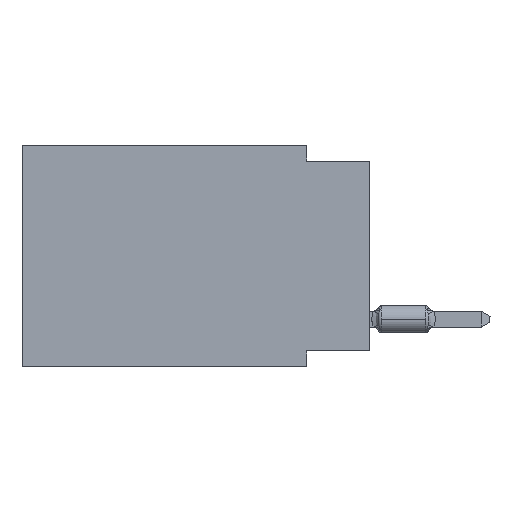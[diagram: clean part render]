
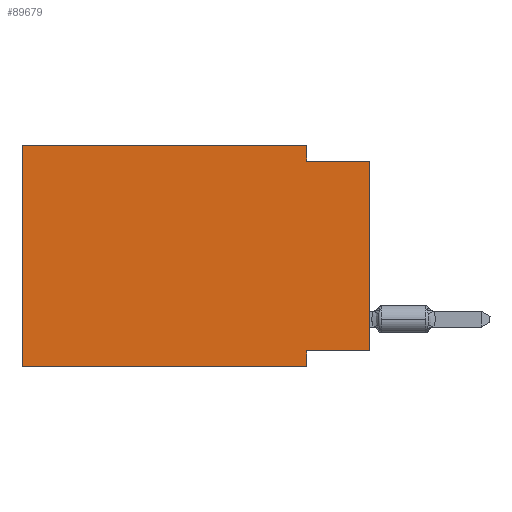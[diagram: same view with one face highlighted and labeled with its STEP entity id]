
A CAD part, left-side view. The second image highlights one B-rep face of the part: STEP entity #89679.
In plain terms, the highlighted planar face has unit normal (-1, 0, 0).
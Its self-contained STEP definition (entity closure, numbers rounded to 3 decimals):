
#3311 = CARTESIAN_POINT ( 'NONE',  ( 0., 2.54, -8.89 ) ) ;
#4840 = CARTESIAN_POINT ( 'NONE',  ( 0., 0., -0.635 ) ) ;
#7582 = PLANE ( 'NONE',  #13161 ) ;
#9186 = ORIENTED_EDGE ( 'NONE', *, *, #81791, .T. ) ;
#12275 = LINE ( 'NONE', #12768, #88802 ) ;
#12284 = DIRECTION ( 'NONE',  ( 0., 0., 1. ) ) ;
#12288 = DIRECTION ( 'NONE',  ( 0., -1., 0. ) ) ;
#12687 = EDGE_LOOP ( 'NONE', ( #56744, #20710, #52912, #78316, #48827, #9186, #57996, #62685 ) ) ;
#12768 = CARTESIAN_POINT ( 'NONE',  ( 0., 2.54, 0. ) ) ;
#13161 = AXIS2_PLACEMENT_3D ( 'NONE', #30740, #92196, #77064 ) ;
#14681 = CARTESIAN_POINT ( 'NONE',  ( 0., 2.54, -8.89 ) ) ;
#15447 = DIRECTION ( 'NONE',  ( 0., 0., 1. ) ) ;
#17630 = EDGE_CURVE ( 'NONE', #24997, #32959, #20441, .T. ) ;
#19634 = CARTESIAN_POINT ( 'NONE',  ( 0., 2.54, -8.255 ) ) ;
#20353 = LINE ( 'NONE', #60130, #80948 ) ;
#20441 = LINE ( 'NONE', #4840, #30726 ) ;
#20710 = ORIENTED_EDGE ( 'NONE', *, *, #17630, .F. ) ;
#22898 = CARTESIAN_POINT ( 'NONE',  ( 0., 13.97, -8.89 ) ) ;
#24997 = VERTEX_POINT ( 'NONE', #66242 ) ;
#30089 = EDGE_CURVE ( 'NONE', #85466, #39073, #93624, .T. ) ;
#30726 = VECTOR ( 'NONE', #97497, 1000. ) ;
#30740 = CARTESIAN_POINT ( 'NONE',  ( 0., 13.97, 0. ) ) ;
#30998 = CARTESIAN_POINT ( 'NONE',  ( 0., 2.54, 0. ) ) ;
#32959 = VERTEX_POINT ( 'NONE', #60547 ) ;
#33958 = VERTEX_POINT ( 'NONE', #3311 ) ;
#34671 = VECTOR ( 'NONE', #15447, 1000. ) ;
#38296 = FACE_OUTER_BOUND ( 'NONE', #12687, .T. ) ;
#39073 = VERTEX_POINT ( 'NONE', #19634 ) ;
#39525 = VECTOR ( 'NONE', #12284, 1000. ) ;
#45466 = EDGE_CURVE ( 'NONE', #39073, #33958, #62005, .T. ) ;
#47656 = LINE ( 'NONE', #70807, #34671 ) ;
#48593 = VECTOR ( 'NONE', #78010, 1000. ) ;
#48827 = ORIENTED_EDGE ( 'NONE', *, *, #71020, .F. ) ;
#52740 = VECTOR ( 'NONE', #60666, 1000. ) ;
#52912 = ORIENTED_EDGE ( 'NONE', *, *, #90291, .F. ) ;
#55741 = EDGE_CURVE ( 'NONE', #61213, #59531, #20353, .T. ) ;
#56744 = ORIENTED_EDGE ( 'NONE', *, *, #79112, .T. ) ;
#57996 = ORIENTED_EDGE ( 'NONE', *, *, #45466, .F. ) ;
#58350 = VERTEX_POINT ( 'NONE', #83361 ) ;
#58634 = CARTESIAN_POINT ( 'NONE',  ( 0., 0., 0. ) ) ;
#59531 = VERTEX_POINT ( 'NONE', #30998 ) ;
#60130 = CARTESIAN_POINT ( 'NONE',  ( 0., 13.97, 0. ) ) ;
#60547 = CARTESIAN_POINT ( 'NONE',  ( 0., 0., -0.635 ) ) ;
#60666 = DIRECTION ( 'NONE',  ( 0., -1., 0. ) ) ;
#61213 = VERTEX_POINT ( 'NONE', #62800 ) ;
#62005 = LINE ( 'NONE', #14681, #72298 ) ;
#62685 = ORIENTED_EDGE ( 'NONE', *, *, #30089, .F. ) ;
#62800 = CARTESIAN_POINT ( 'NONE',  ( 0., 13.97, 0. ) ) ;
#66242 = CARTESIAN_POINT ( 'NONE',  ( 0., 2.54, -0.635 ) ) ;
#70210 = LINE ( 'NONE', #22898, #52740 ) ;
#70807 = CARTESIAN_POINT ( 'NONE',  ( 0., 13.97, 0. ) ) ;
#71020 = EDGE_CURVE ( 'NONE', #58350, #61213, #47656, .T. ) ;
#72298 = VECTOR ( 'NONE', #84665, 1000. ) ;
#77064 = DIRECTION ( 'NONE',  ( 0., 0., -1. ) ) ;
#78010 = DIRECTION ( 'NONE',  ( 0., 1., 0. ) ) ;
#78316 = ORIENTED_EDGE ( 'NONE', *, *, #55741, .F. ) ;
#79112 = EDGE_CURVE ( 'NONE', #85466, #32959, #81295, .T. ) ;
#80948 = VECTOR ( 'NONE', #12288, 1000. ) ;
#81287 = DIRECTION ( 'NONE',  ( 0., 0., -1. ) ) ;
#81295 = LINE ( 'NONE', #58634, #39525 ) ;
#81791 = EDGE_CURVE ( 'NONE', #58350, #33958, #70210, .T. ) ;
#83361 = CARTESIAN_POINT ( 'NONE',  ( 0., 13.97, -8.89 ) ) ;
#84082 = CARTESIAN_POINT ( 'NONE',  ( 0., 0., -8.255 ) ) ;
#84665 = DIRECTION ( 'NONE',  ( 0., 0., -1. ) ) ;
#85466 = VERTEX_POINT ( 'NONE', #87436 ) ;
#87436 = CARTESIAN_POINT ( 'NONE',  ( 0., 0., -8.255 ) ) ;
#88802 = VECTOR ( 'NONE', #81287, 1000. ) ;
#89679 = ADVANCED_FACE ( 'NONE', ( #38296 ), #7582, .F. ) ;
#90291 = EDGE_CURVE ( 'NONE', #59531, #24997, #12275, .T. ) ;
#92196 = DIRECTION ( 'NONE',  ( 1., 0., 0. ) ) ;
#93624 = LINE ( 'NONE', #84082, #48593 ) ;
#97497 = DIRECTION ( 'NONE',  ( 0., -1., 0. ) ) ;
